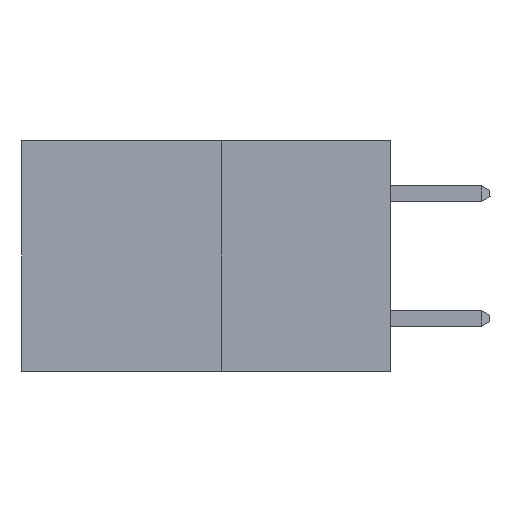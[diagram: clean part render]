
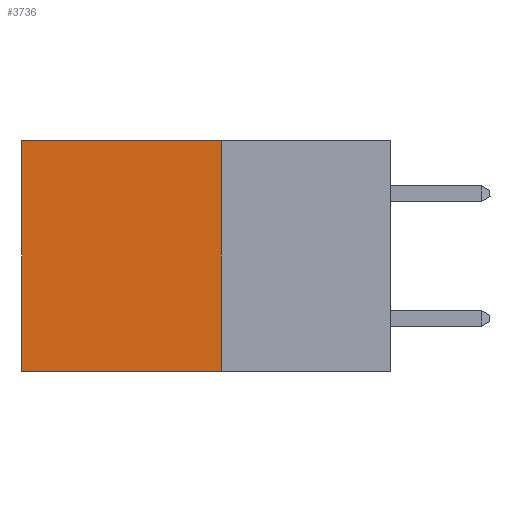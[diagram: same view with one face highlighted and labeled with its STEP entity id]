
A CAD part, left-side view. The second image highlights one B-rep face of the part: STEP entity #3736.
In plain terms, the highlighted planar face has unit normal (-1, 0, 0).
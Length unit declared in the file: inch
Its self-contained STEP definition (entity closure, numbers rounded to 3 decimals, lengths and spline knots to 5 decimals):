
#292 = CARTESIAN_POINT ( 'NONE',  ( 0.277, 0.27, 0. ) ) ;
#593 = EDGE_CURVE ( 'NONE', #4852, #6479, #2538, .T. ) ;
#2280 = CARTESIAN_POINT ( 'NONE',  ( 0.277, 0.27, -0.37 ) ) ;
#2538 = LINE ( 'NONE', #12294, #2982 ) ;
#2982 = VECTOR ( 'NONE', #11088, 39.37008 ) ;
#3683 = VECTOR ( 'NONE', #14817, 39.37008 ) ;
#3736 = ADVANCED_FACE ( 'NONE', ( #11460 ), #12212, .F. ) ;
#4852 = VERTEX_POINT ( 'NONE', #12366 ) ;
#6058 = DIRECTION ( 'NONE',  ( 1., 0., 0. ) ) ;
#6479 = VERTEX_POINT ( 'NONE', #2280 ) ;
#6598 = EDGE_CURVE ( 'NONE', #6479, #12257, #6732, .T. ) ;
#6732 = LINE ( 'NONE', #10754, #11534 ) ;
#7100 = ORIENTED_EDGE ( 'NONE', *, *, #6598, .F. ) ;
#7155 = ORIENTED_EDGE ( 'NONE', *, *, #10988, .T. ) ;
#7515 = VECTOR ( 'NONE', #13268, 39.37008 ) ;
#8091 = DIRECTION ( 'NONE',  ( 0., 0., -1. ) ) ;
#8277 = VERTEX_POINT ( 'NONE', #15606 ) ;
#8780 = CARTESIAN_POINT ( 'NONE',  ( 0.277, 0.59, -0.37 ) ) ;
#9011 = EDGE_CURVE ( 'NONE', #4852, #8277, #15255, .T. ) ;
#9059 = ORIENTED_EDGE ( 'NONE', *, *, #9011, .T. ) ;
#10003 = CARTESIAN_POINT ( 'NONE',  ( 0.277, 0.59, -0.37 ) ) ;
#10384 = DIRECTION ( 'NONE',  ( 0., 1., 0. ) ) ;
#10754 = CARTESIAN_POINT ( 'NONE',  ( 0.277, 0.27, -0.37 ) ) ;
#10988 = EDGE_CURVE ( 'NONE', #8277, #12257, #11470, .T. ) ;
#11088 = DIRECTION ( 'NONE',  ( 0., 0., -1. ) ) ;
#11460 = FACE_OUTER_BOUND ( 'NONE', #18342, .T. ) ;
#11470 = LINE ( 'NONE', #10003, #3683 ) ;
#11534 = VECTOR ( 'NONE', #10384, 39.37008 ) ;
#12212 = PLANE ( 'NONE',  #18181 ) ;
#12257 = VERTEX_POINT ( 'NONE', #8780 ) ;
#12294 = CARTESIAN_POINT ( 'NONE',  ( 0.277, 0.27, -0.37 ) ) ;
#12366 = CARTESIAN_POINT ( 'NONE',  ( 0.277, 0.27, 0. ) ) ;
#13268 = DIRECTION ( 'NONE',  ( 0., 1., 0. ) ) ;
#14020 = CARTESIAN_POINT ( 'NONE',  ( 0.277, 0.27, -0.37 ) ) ;
#14817 = DIRECTION ( 'NONE',  ( 0., 0., -1. ) ) ;
#15255 = LINE ( 'NONE', #292, #7515 ) ;
#15606 = CARTESIAN_POINT ( 'NONE',  ( 0.277, 0.59, 0. ) ) ;
#15611 = ORIENTED_EDGE ( 'NONE', *, *, #593, .F. ) ;
#18181 = AXIS2_PLACEMENT_3D ( 'NONE', #14020, #6058, #8091 ) ;
#18342 = EDGE_LOOP ( 'NONE', ( #7155, #7100, #15611, #9059 ) ) ;
